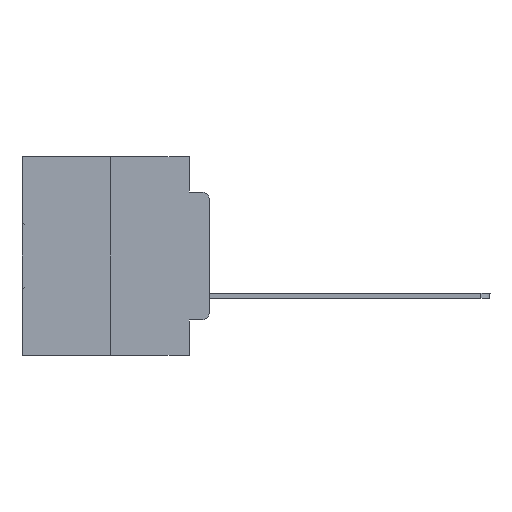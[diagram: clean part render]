
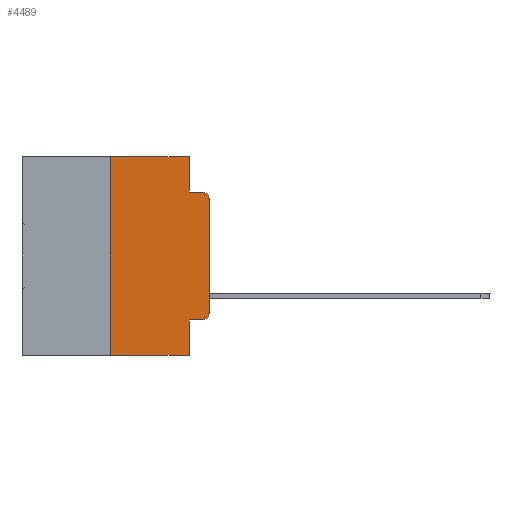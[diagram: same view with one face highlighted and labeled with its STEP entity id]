
A CAD part, left-side view. The second image highlights one B-rep face of the part: STEP entity #4489.
In plain terms, the highlighted planar face has unit normal (-1, 0, 0).
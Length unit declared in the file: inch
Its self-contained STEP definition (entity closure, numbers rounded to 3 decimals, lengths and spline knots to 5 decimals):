
#627 = EDGE_LOOP ( 'NONE', ( #18507, #24216, #959, #29969, #10166, #23064, #27891, #24325, #4810, #23571 ) ) ;
#659 = VECTOR ( 'NONE', #11337, 39.37008 ) ;
#766 = CARTESIAN_POINT ( 'NONE',  ( 0., 0., 0. ) ) ;
#959 = ORIENTED_EDGE ( 'NONE', *, *, #12975, .F. ) ;
#1220 = VECTOR ( 'NONE', #19453, 39.37008 ) ;
#1476 = CIRCLE ( 'NONE', #3908, 0.02 ) ;
#1645 = CARTESIAN_POINT ( 'NONE',  ( 0., 0.473, 0. ) ) ;
#1899 = DIRECTION ( 'NONE',  ( 0., -1., 0. ) ) ;
#2302 = CARTESIAN_POINT ( 'NONE',  ( 0., 0.02, -0.1085 ) ) ;
#2598 = CARTESIAN_POINT ( 'NONE',  ( 0., 0.02, -0.0885 ) ) ;
#2706 = LINE ( 'NONE', #29639, #30777 ) ;
#3494 = CARTESIAN_POINT ( 'NONE',  ( 0., 0.051, 0. ) ) ;
#3656 = EDGE_CURVE ( 'NONE', #21030, #25747, #28905, .T. ) ;
#3908 = AXIS2_PLACEMENT_3D ( 'NONE', #29431, #24320, #9447 ) ;
#4290 = DIRECTION ( 'NONE',  ( 0., -1., 0. ) ) ;
#4489 = ADVANCED_FACE ( 'NONE', ( #28475 ), #32440, .F. ) ;
#4810 = ORIENTED_EDGE ( 'NONE', *, *, #12651, .T. ) ;
#5083 = DIRECTION ( 'NONE',  ( -1., 0., 0. ) ) ;
#7555 = CARTESIAN_POINT ( 'NONE',  ( 0., 0.02, -0.4115 ) ) ;
#8108 = CARTESIAN_POINT ( 'NONE',  ( 0., 0.051, 0. ) ) ;
#8380 = LINE ( 'NONE', #8108, #12357 ) ;
#8563 = CARTESIAN_POINT ( 'NONE',  ( 0., 0.051, -0.4115 ) ) ;
#8707 = VERTEX_POINT ( 'NONE', #21345 ) ;
#9021 = LINE ( 'NONE', #3494, #659 ) ;
#9330 = EDGE_CURVE ( 'NONE', #21232, #20349, #1476, .T. ) ;
#9447 = DIRECTION ( 'NONE',  ( 0., 0., -1. ) ) ;
#9976 = CIRCLE ( 'NONE', #18264, 0.02 ) ;
#10052 = DIRECTION ( 'NONE',  ( 0., 0., -1. ) ) ;
#10166 = ORIENTED_EDGE ( 'NONE', *, *, #3656, .F. ) ;
#11177 = CARTESIAN_POINT ( 'NONE',  ( 0., 0.25, 0. ) ) ;
#11337 = DIRECTION ( 'NONE',  ( 0., 0., -1. ) ) ;
#11997 = VERTEX_POINT ( 'NONE', #12107 ) ;
#12107 = CARTESIAN_POINT ( 'NONE',  ( 0., 0.25, -0.5 ) ) ;
#12357 = VECTOR ( 'NONE', #30994, 39.37008 ) ;
#12651 = EDGE_CURVE ( 'NONE', #16307, #21232, #12750, .T. ) ;
#12750 = LINE ( 'NONE', #19413, #27375 ) ;
#12975 = EDGE_CURVE ( 'NONE', #8707, #15771, #26567, .T. ) ;
#14498 = DIRECTION ( 'NONE',  ( 0., -1., 0. ) ) ;
#15771 = VERTEX_POINT ( 'NONE', #2598 ) ;
#16274 = EDGE_CURVE ( 'NONE', #16307, #16279, #9021, .T. ) ;
#16279 = VERTEX_POINT ( 'NONE', #23574 ) ;
#16307 = VERTEX_POINT ( 'NONE', #8563 ) ;
#16886 = LINE ( 'NONE', #766, #29535 ) ;
#16903 = AXIS2_PLACEMENT_3D ( 'NONE', #22265, #19517, #29441 ) ;
#17364 = CARTESIAN_POINT ( 'NONE',  ( 0., 0.051, -0.0885 ) ) ;
#17514 = CARTESIAN_POINT ( 'NONE',  ( 0., 0.051, 0. ) ) ;
#18264 = AXIS2_PLACEMENT_3D ( 'NONE', #2302, #5083, #10052 ) ;
#18507 = ORIENTED_EDGE ( 'NONE', *, *, #28904, .T. ) ;
#19007 = DIRECTION ( 'NONE',  ( 0., 0., 1. ) ) ;
#19413 = CARTESIAN_POINT ( 'NONE',  ( 0., 0.051, -0.4115 ) ) ;
#19453 = DIRECTION ( 'NONE',  ( 0., -1., 0. ) ) ;
#19517 = DIRECTION ( 'NONE',  ( 1., 0., 0. ) ) ;
#19877 = VECTOR ( 'NONE', #1899, 39.37008 ) ;
#20349 = VERTEX_POINT ( 'NONE', #24382 ) ;
#20470 = EDGE_CURVE ( 'NONE', #23981, #15771, #9976, .T. ) ;
#20496 = CARTESIAN_POINT ( 'NONE',  ( 0., 0., -0.1085 ) ) ;
#21030 = VERTEX_POINT ( 'NONE', #32560 ) ;
#21232 = VERTEX_POINT ( 'NONE', #7555 ) ;
#21345 = CARTESIAN_POINT ( 'NONE',  ( 0., 0.051, -0.0885 ) ) ;
#21619 = LINE ( 'NONE', #11177, #27921 ) ;
#22265 = CARTESIAN_POINT ( 'NONE',  ( 0., 0.473, 0. ) ) ;
#23064 = ORIENTED_EDGE ( 'NONE', *, *, #29046, .F. ) ;
#23414 = DIRECTION ( 'NONE',  ( 0., 0., 1. ) ) ;
#23571 = ORIENTED_EDGE ( 'NONE', *, *, #9330, .T. ) ;
#23574 = CARTESIAN_POINT ( 'NONE',  ( 0., 0.051, -0.5 ) ) ;
#23981 = VERTEX_POINT ( 'NONE', #20496 ) ;
#24216 = ORIENTED_EDGE ( 'NONE', *, *, #20470, .T. ) ;
#24320 = DIRECTION ( 'NONE',  ( -1., 0., 0. ) ) ;
#24325 = ORIENTED_EDGE ( 'NONE', *, *, #16274, .F. ) ;
#24382 = CARTESIAN_POINT ( 'NONE',  ( 0., 0., -0.3915 ) ) ;
#25747 = VERTEX_POINT ( 'NONE', #17514 ) ;
#26567 = LINE ( 'NONE', #17364, #19877 ) ;
#27375 = VECTOR ( 'NONE', #4290, 39.37008 ) ;
#27891 = ORIENTED_EDGE ( 'NONE', *, *, #28121, .T. ) ;
#27921 = VECTOR ( 'NONE', #19007, 39.37008 ) ;
#28121 = EDGE_CURVE ( 'NONE', #11997, #16279, #2706, .T. ) ;
#28475 = FACE_OUTER_BOUND ( 'NONE', #627, .T. ) ;
#28904 = EDGE_CURVE ( 'NONE', #20349, #23981, #16886, .T. ) ;
#28905 = LINE ( 'NONE', #1645, #1220 ) ;
#29046 = EDGE_CURVE ( 'NONE', #11997, #21030, #21619, .T. ) ;
#29431 = CARTESIAN_POINT ( 'NONE',  ( 0., 0.02, -0.3915 ) ) ;
#29441 = DIRECTION ( 'NONE',  ( 0., 0., -1. ) ) ;
#29535 = VECTOR ( 'NONE', #23414, 39.37008 ) ;
#29639 = CARTESIAN_POINT ( 'NONE',  ( 0., 0.473, -0.5 ) ) ;
#29969 = ORIENTED_EDGE ( 'NONE', *, *, #32039, .F. ) ;
#30777 = VECTOR ( 'NONE', #14498, 39.37008 ) ;
#30994 = DIRECTION ( 'NONE',  ( 0., 0., -1. ) ) ;
#32039 = EDGE_CURVE ( 'NONE', #25747, #8707, #8380, .T. ) ;
#32440 = PLANE ( 'NONE',  #16903 ) ;
#32560 = CARTESIAN_POINT ( 'NONE',  ( 0., 0.25, 0. ) ) ;
